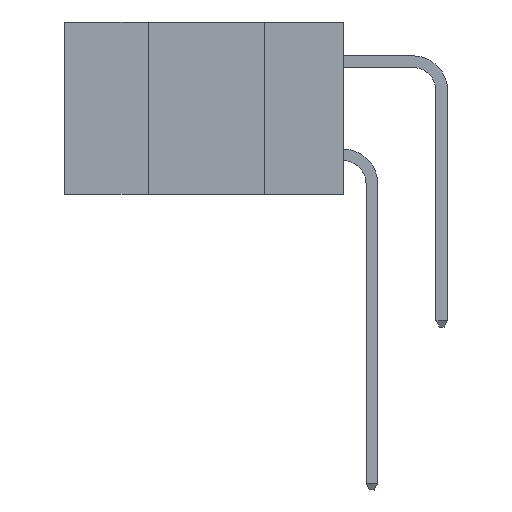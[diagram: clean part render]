
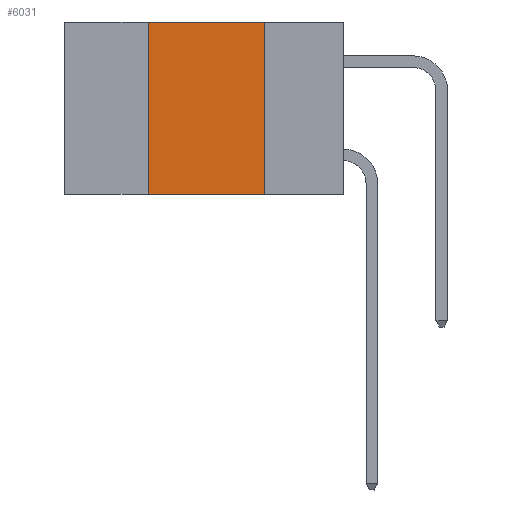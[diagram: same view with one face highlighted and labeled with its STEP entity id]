
A CAD part, left-side view. The second image highlights one B-rep face of the part: STEP entity #6031.
In plain terms, the highlighted planar face has unit normal (-1, 0, 0).
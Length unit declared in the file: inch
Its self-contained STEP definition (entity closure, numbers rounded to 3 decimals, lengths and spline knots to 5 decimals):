
#77 = DIRECTION ( 'NONE',  ( 1., 0., 0. ) ) ;
#254 = DIRECTION ( 'NONE',  ( 0., 0., -1. ) ) ;
#548 = PLANE ( 'NONE',  #12611 ) ;
#901 = DIRECTION ( 'NONE',  ( 0., 0., 1. ) ) ;
#1003 = LINE ( 'NONE', #1871, #5898 ) ;
#1220 = VECTOR ( 'NONE', #8244, 39.37008 ) ;
#1539 = LINE ( 'NONE', #8632, #1220 ) ;
#1605 = CARTESIAN_POINT ( 'NONE',  ( 0., 0.6, 0. ) ) ;
#1634 = EDGE_CURVE ( 'NONE', #9443, #9274, #12073, .T. ) ;
#1871 = CARTESIAN_POINT ( 'NONE',  ( 0., 0.6, 0. ) ) ;
#2842 = DIRECTION ( 'NONE',  ( 0., -1., 0. ) ) ;
#3011 = LINE ( 'NONE', #13059, #7698 ) ;
#3077 = CARTESIAN_POINT ( 'NONE',  ( 0., 0.42, 0. ) ) ;
#3581 = VECTOR ( 'NONE', #3898, 39.37008 ) ;
#3603 = CARTESIAN_POINT ( 'NONE',  ( 0., 0.6, -0.37 ) ) ;
#3898 = DIRECTION ( 'NONE',  ( 0., -1., 0. ) ) ;
#4381 = ORIENTED_EDGE ( 'NONE', *, *, #7732, .F. ) ;
#4871 = CARTESIAN_POINT ( 'NONE',  ( 0., 0.17, 0. ) ) ;
#4953 = EDGE_CURVE ( 'NONE', #11134, #9274, #1539, .T. ) ;
#5898 = VECTOR ( 'NONE', #2842, 39.37008 ) ;
#6031 = ADVANCED_FACE ( 'NONE', ( #9382 ), #548, .F. ) ;
#6477 = ORIENTED_EDGE ( 'NONE', *, *, #1634, .T. ) ;
#7099 = EDGE_CURVE ( 'NONE', #9443, #12918, #3011, .T. ) ;
#7698 = VECTOR ( 'NONE', #901, 39.37008 ) ;
#7732 = EDGE_CURVE ( 'NONE', #12918, #11134, #1003, .T. ) ;
#7840 = CARTESIAN_POINT ( 'NONE',  ( 0., 0.17, -0.37 ) ) ;
#8244 = DIRECTION ( 'NONE',  ( 0., 0., -1. ) ) ;
#8632 = CARTESIAN_POINT ( 'NONE',  ( 0., 0.17, 0. ) ) ;
#8656 = EDGE_LOOP ( 'NONE', ( #8781, #4381, #9748, #6477 ) ) ;
#8781 = ORIENTED_EDGE ( 'NONE', *, *, #4953, .F. ) ;
#9274 = VERTEX_POINT ( 'NONE', #7840 ) ;
#9382 = FACE_OUTER_BOUND ( 'NONE', #8656, .T. ) ;
#9443 = VERTEX_POINT ( 'NONE', #10155 ) ;
#9748 = ORIENTED_EDGE ( 'NONE', *, *, #7099, .F. ) ;
#10155 = CARTESIAN_POINT ( 'NONE',  ( 0., 0.42, -0.37 ) ) ;
#11134 = VERTEX_POINT ( 'NONE', #4871 ) ;
#12073 = LINE ( 'NONE', #3603, #3581 ) ;
#12611 = AXIS2_PLACEMENT_3D ( 'NONE', #1605, #77, #254 ) ;
#12918 = VERTEX_POINT ( 'NONE', #3077 ) ;
#13059 = CARTESIAN_POINT ( 'NONE',  ( 0., 0.42, 0. ) ) ;
